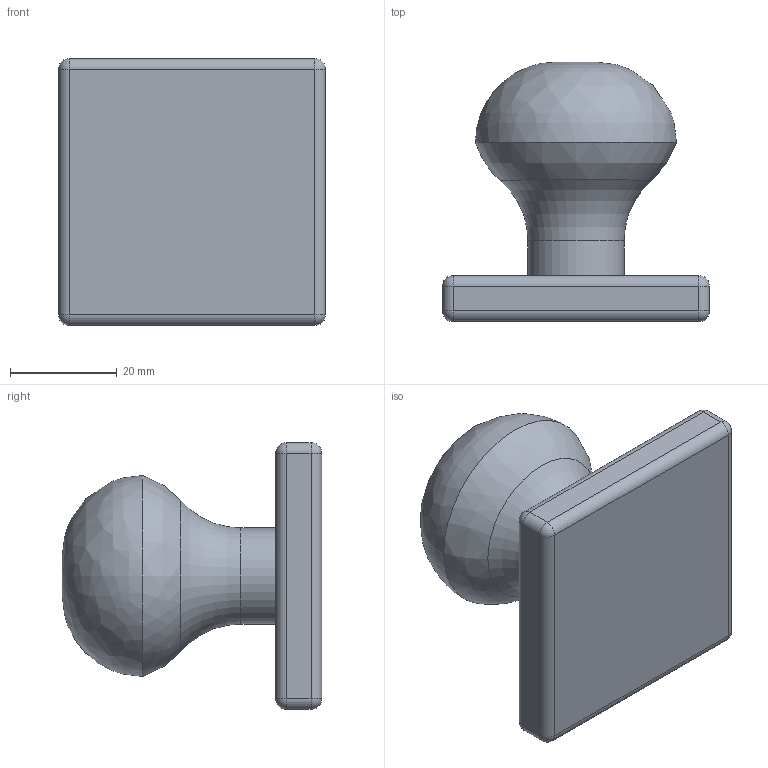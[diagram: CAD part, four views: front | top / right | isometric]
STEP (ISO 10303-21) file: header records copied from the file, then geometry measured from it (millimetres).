
FILE_DESCRIPTION(/* description */ (''),/* implementation_level */ '2;1');
FILE_NAME(/* name */ 'freeman1337-ar15-speedloader-pusher.step',/* time_stamp */ '2021-08-30T09:56:17-07:00',/* author */ (''),/* organization */ (''),/* preprocessor_version */ 'ST-DEVELOPER v18.1',/* originating_system */ 'Autodesk Translation Framework v10.10.0.1391',/* authorisation */ '');
FILE_SCHEMA (('AUTOMOTIVE_DESIGN { 1 0 10303 214 3 1 1 }'));
Length unit declared in the file: millimetre
Products named in the file (1): pusher (1)
Bounding box: 50 x 48.6 x 50 mm (x, y, z)
Volume: 45393.9 mm3; surface area: 10267.9 mm2
Topology: 1 solids, 1 shells, 31 faces, 58 edges, 30 vertices
Faces by surface type: cylinder 13, sphere 8, plane 7, bspline 2, torus 1
Full cylindrical faces by diameter (mm): 18 x1
Entity records: 834 total; most frequent: CARTESIAN_POINT 172, DIRECTION 151, ORIENTED_EDGE 116, AXIS2_PLACEMENT_3D 63, EDGE_CURVE 58, CIRCLE 33, EDGE_LOOP 32, FACE_OUTER_BOUND 31
